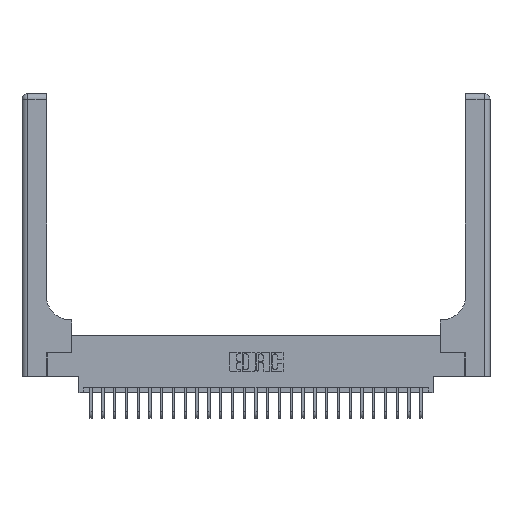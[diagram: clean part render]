
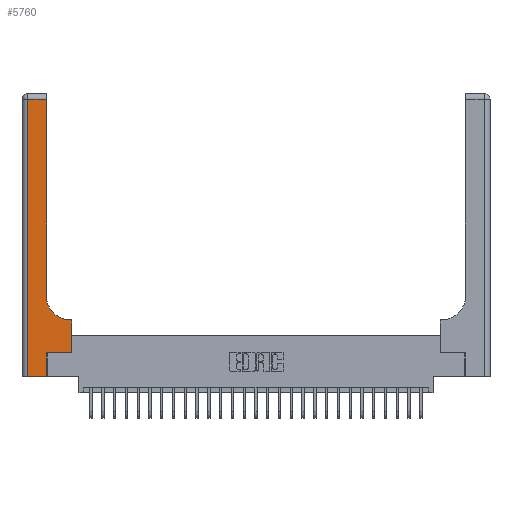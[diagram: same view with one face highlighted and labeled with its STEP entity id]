
A CAD part, top view. The second image highlights one B-rep face of the part: STEP entity #5760.
In plain terms, the highlighted planar face has unit normal (0, 0, 1).
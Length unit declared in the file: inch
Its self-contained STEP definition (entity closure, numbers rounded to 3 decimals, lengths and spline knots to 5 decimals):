
#132 = DIRECTION ( 'NONE',  ( 1., 0., 0. ) ) ;
#503 = VERTEX_POINT ( 'NONE', #24788 ) ;
#744 = EDGE_CURVE ( 'NONE', #18519, #2638, #25386, .T. ) ;
#923 = CARTESIAN_POINT ( 'NONE',  ( 0., 2.94, 0.37 ) ) ;
#1171 = CARTESIAN_POINT ( 'NONE',  ( 0.06, 3., 0.37 ) ) ;
#1428 = LINE ( 'NONE', #17191, #13890 ) ;
#1536 = DIRECTION ( 'NONE',  ( -1., 0., 0. ) ) ;
#1915 = CIRCLE ( 'NONE', #8372, 0.25 ) ;
#2638 = VERTEX_POINT ( 'NONE', #18599 ) ;
#3256 = VECTOR ( 'NONE', #5212, 39.37008 ) ;
#3744 = EDGE_CURVE ( 'NONE', #503, #17602, #1428, .T. ) ;
#5119 = CARTESIAN_POINT ( 'NONE',  ( 0.528, 0.6, 0.37 ) ) ;
#5212 = DIRECTION ( 'NONE',  ( -1., 0., 0. ) ) ;
#5539 = LINE ( 'NONE', #15207, #12289 ) ;
#5581 = VERTEX_POINT ( 'NONE', #22192 ) ;
#5599 = ORIENTED_EDGE ( 'NONE', *, *, #3744, .T. ) ;
#5760 = ADVANCED_FACE ( 'NONE', ( #13816 ), #22583, .F. ) ;
#5925 = LINE ( 'NONE', #923, #3256 ) ;
#6635 = ORIENTED_EDGE ( 'NONE', *, *, #25218, .T. ) ;
#7109 = ORIENTED_EDGE ( 'NONE', *, *, #25129, .T. ) ;
#7227 = ORIENTED_EDGE ( 'NONE', *, *, #744, .T. ) ;
#7915 = VERTEX_POINT ( 'NONE', #17143 ) ;
#8372 = AXIS2_PLACEMENT_3D ( 'NONE', #8860, #25826, #132 ) ;
#8619 = VECTOR ( 'NONE', #20723, 39.37008 ) ;
#8860 = CARTESIAN_POINT ( 'NONE',  ( 0.51, 0.85, 0.37 ) ) ;
#9595 = EDGE_CURVE ( 'NONE', #18438, #5581, #9618, .T. ) ;
#9618 = LINE ( 'NONE', #27026, #8619 ) ;
#9742 = CARTESIAN_POINT ( 'NONE',  ( 0., 3., 0.37 ) ) ;
#9867 = EDGE_CURVE ( 'NONE', #13407, #7915, #5539, .T. ) ;
#10904 = ORIENTED_EDGE ( 'NONE', *, *, #18935, .T. ) ;
#11445 = EDGE_CURVE ( 'NONE', #13742, #18438, #19910, .T. ) ;
#11692 = CARTESIAN_POINT ( 'NONE',  ( 0.265, 0., 0.37 ) ) ;
#12207 = VECTOR ( 'NONE', #20598, 39.37008 ) ;
#12289 = VECTOR ( 'NONE', #12888, 39.37008 ) ;
#12295 = CARTESIAN_POINT ( 'NONE',  ( 0.528, 0.25, 0.37 ) ) ;
#12888 = DIRECTION ( 'NONE',  ( 0., 1., 0. ) ) ;
#13407 = VERTEX_POINT ( 'NONE', #16491 ) ;
#13668 = EDGE_LOOP ( 'NONE', ( #14238, #14724, #25575, #23371, #6635, #5599, #7109, #7227, #10904 ) ) ;
#13742 = VERTEX_POINT ( 'NONE', #17978 ) ;
#13816 = FACE_OUTER_BOUND ( 'NONE', #13668, .T. ) ;
#13890 = VECTOR ( 'NONE', #25441, 39.37008 ) ;
#14238 = ORIENTED_EDGE ( 'NONE', *, *, #9867, .T. ) ;
#14472 = LINE ( 'NONE', #11692, #18488 ) ;
#14527 = DIRECTION ( 'NONE',  ( 0., 0., -1. ) ) ;
#14724 = ORIENTED_EDGE ( 'NONE', *, *, #19810, .T. ) ;
#15018 = CARTESIAN_POINT ( 'NONE',  ( 0.06, 0., 0.37 ) ) ;
#15207 = CARTESIAN_POINT ( 'NONE',  ( 0.26, 3., 0.37 ) ) ;
#16491 = CARTESIAN_POINT ( 'NONE',  ( 0.26, 0.85, 0.37 ) ) ;
#17143 = CARTESIAN_POINT ( 'NONE',  ( 0.26, 2.94, 0.37 ) ) ;
#17191 = CARTESIAN_POINT ( 'NONE',  ( 0.265, 0.25, 0.37 ) ) ;
#17602 = VERTEX_POINT ( 'NONE', #12295 ) ;
#17968 = DIRECTION ( 'NONE',  ( 0., 1., 0. ) ) ;
#17978 = CARTESIAN_POINT ( 'NONE',  ( 0.06, 2.94, 0.37 ) ) ;
#18438 = VERTEX_POINT ( 'NONE', #15018 ) ;
#18488 = VECTOR ( 'NONE', #26593, 39.37008 ) ;
#18519 = VERTEX_POINT ( 'NONE', #5119 ) ;
#18599 = CARTESIAN_POINT ( 'NONE',  ( 0.51, 0.6, 0.37 ) ) ;
#18797 = LINE ( 'NONE', #24129, #20165 ) ;
#18935 = EDGE_CURVE ( 'NONE', #2638, #13407, #1915, .T. ) ;
#19686 = VECTOR ( 'NONE', #23823, 39.37008 ) ;
#19810 = EDGE_CURVE ( 'NONE', #7915, #13742, #5925, .T. ) ;
#19910 = LINE ( 'NONE', #1171, #12207 ) ;
#20165 = VECTOR ( 'NONE', #17968, 39.37008 ) ;
#20598 = DIRECTION ( 'NONE',  ( 0., -1., 0. ) ) ;
#20723 = DIRECTION ( 'NONE',  ( 1., 0., 0. ) ) ;
#22192 = CARTESIAN_POINT ( 'NONE',  ( 0.265, 0., 0.37 ) ) ;
#22583 = PLANE ( 'NONE',  #25808 ) ;
#23371 = ORIENTED_EDGE ( 'NONE', *, *, #9595, .T. ) ;
#23823 = DIRECTION ( 'NONE',  ( -1., 0., 0. ) ) ;
#24129 = CARTESIAN_POINT ( 'NONE',  ( 0.528, 0.25, 0.37 ) ) ;
#24788 = CARTESIAN_POINT ( 'NONE',  ( 0.265, 0.25, 0.37 ) ) ;
#25129 = EDGE_CURVE ( 'NONE', #17602, #18519, #18797, .T. ) ;
#25218 = EDGE_CURVE ( 'NONE', #5581, #503, #14472, .T. ) ;
#25386 = LINE ( 'NONE', #25805, #19686 ) ;
#25441 = DIRECTION ( 'NONE',  ( 1., 0., 0. ) ) ;
#25575 = ORIENTED_EDGE ( 'NONE', *, *, #11445, .T. ) ;
#25805 = CARTESIAN_POINT ( 'NONE',  ( 0.26, 0.6, 0.37 ) ) ;
#25808 = AXIS2_PLACEMENT_3D ( 'NONE', #9742, #14527, #1536 ) ;
#25826 = DIRECTION ( 'NONE',  ( 0., 0., -1. ) ) ;
#26593 = DIRECTION ( 'NONE',  ( 0., 1., 0. ) ) ;
#27026 = CARTESIAN_POINT ( 'NONE',  ( 0., 0., 0.37 ) ) ;
